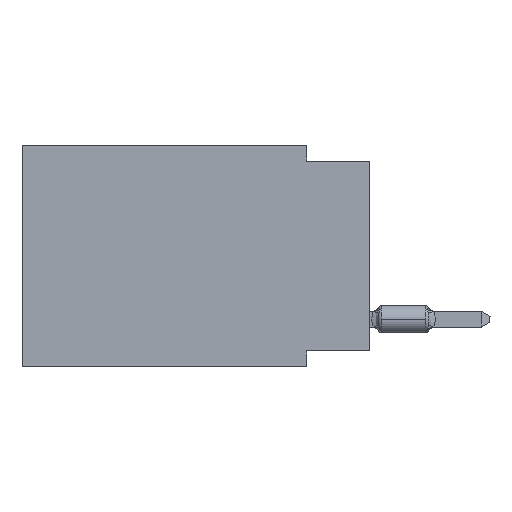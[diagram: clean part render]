
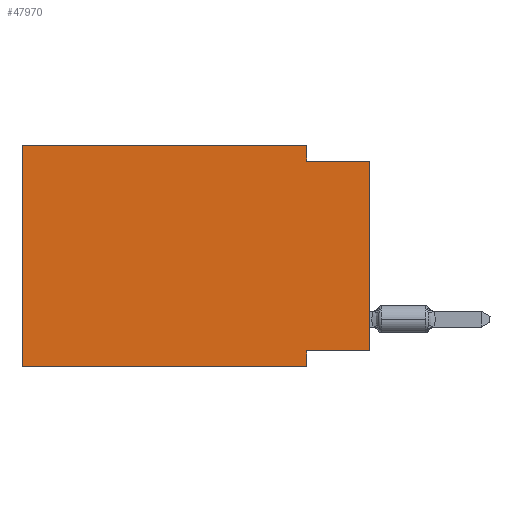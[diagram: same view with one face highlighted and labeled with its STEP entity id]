
A CAD part, left-side view. The second image highlights one B-rep face of the part: STEP entity #47970.
In plain terms, the highlighted planar face has unit normal (-1, 0, 0).
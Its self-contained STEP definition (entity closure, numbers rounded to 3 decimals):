
#74 = EDGE_CURVE ( 'NONE', #14920, #34732, #71550, .T. ) ;
#861 = CARTESIAN_POINT ( 'NONE',  ( 0., 0., -8.255 ) ) ;
#1129 = VERTEX_POINT ( 'NONE', #37625 ) ;
#1969 = LINE ( 'NONE', #44744, #39972 ) ;
#2510 = VERTEX_POINT ( 'NONE', #58885 ) ;
#4873 = LINE ( 'NONE', #11194, #41778 ) ;
#4916 = ORIENTED_EDGE ( 'NONE', *, *, #40327, .F. ) ;
#5290 = ORIENTED_EDGE ( 'NONE', *, *, #49267, .F. ) ;
#5528 = VECTOR ( 'NONE', #20194, 1000. ) ;
#7954 = VECTOR ( 'NONE', #27954, 1000. ) ;
#8227 = DIRECTION ( 'NONE',  ( 0., 0., -1. ) ) ;
#8551 = EDGE_CURVE ( 'NONE', #14920, #77421, #48816, .T. ) ;
#10298 = VECTOR ( 'NONE', #41719, 1000. ) ;
#11194 = CARTESIAN_POINT ( 'NONE',  ( 0., 0., -0.635 ) ) ;
#11829 = DIRECTION ( 'NONE',  ( 0., 0., -1. ) ) ;
#12386 = VERTEX_POINT ( 'NONE', #71640 ) ;
#14219 = LINE ( 'NONE', #50292, #5528 ) ;
#14920 = VERTEX_POINT ( 'NONE', #39695 ) ;
#15002 = ORIENTED_EDGE ( 'NONE', *, *, #8551, .F. ) ;
#16482 = CARTESIAN_POINT ( 'NONE',  ( 0., 2.54, -8.255 ) ) ;
#17542 = ORIENTED_EDGE ( 'NONE', *, *, #74, .T. ) ;
#18570 = PLANE ( 'NONE',  #43942 ) ;
#19170 = ORIENTED_EDGE ( 'NONE', *, *, #73306, .F. ) ;
#20041 = VECTOR ( 'NONE', #8227, 1000. ) ;
#20194 = DIRECTION ( 'NONE',  ( 0., 0., 1. ) ) ;
#20513 = CARTESIAN_POINT ( 'NONE',  ( 0., 2.54, 0. ) ) ;
#21476 = ORIENTED_EDGE ( 'NONE', *, *, #29400, .F. ) ;
#25407 = CARTESIAN_POINT ( 'NONE',  ( 0., 13.97, -8.89 ) ) ;
#27954 = DIRECTION ( 'NONE',  ( 0., 0., 1. ) ) ;
#29272 = DIRECTION ( 'NONE',  ( 1., 0., 0. ) ) ;
#29400 = EDGE_CURVE ( 'NONE', #1129, #34732, #4873, .T. ) ;
#34732 = VERTEX_POINT ( 'NONE', #48716 ) ;
#37157 = LINE ( 'NONE', #20513, #20041 ) ;
#37416 = VERTEX_POINT ( 'NONE', #25407 ) ;
#37551 = LINE ( 'NONE', #56172, #40257 ) ;
#37625 = CARTESIAN_POINT ( 'NONE',  ( 0., 2.54, -0.635 ) ) ;
#39207 = DIRECTION ( 'NONE',  ( 0., -1., 0. ) ) ;
#39381 = ORIENTED_EDGE ( 'NONE', *, *, #46303, .F. ) ;
#39695 = CARTESIAN_POINT ( 'NONE',  ( 0., 0., -8.255 ) ) ;
#39972 = VECTOR ( 'NONE', #63002, 1000. ) ;
#40257 = VECTOR ( 'NONE', #61752, 1000. ) ;
#40327 = EDGE_CURVE ( 'NONE', #2510, #1129, #37157, .T. ) ;
#41719 = DIRECTION ( 'NONE',  ( 0., 1., 0. ) ) ;
#41778 = VECTOR ( 'NONE', #59547, 1000. ) ;
#41809 = CARTESIAN_POINT ( 'NONE',  ( 0., 0., 0. ) ) ;
#42128 = CARTESIAN_POINT ( 'NONE',  ( 0., 13.97, 0. ) ) ;
#43942 = AXIS2_PLACEMENT_3D ( 'NONE', #47899, #29272, #11829 ) ;
#44744 = CARTESIAN_POINT ( 'NONE',  ( 0., 13.97, 0. ) ) ;
#46303 = EDGE_CURVE ( 'NONE', #53779, #2510, #1969, .T. ) ;
#47899 = CARTESIAN_POINT ( 'NONE',  ( 0., 13.97, 0. ) ) ;
#47970 = ADVANCED_FACE ( 'NONE', ( #78053 ), #18570, .F. ) ;
#48716 = CARTESIAN_POINT ( 'NONE',  ( 0., 0., -0.635 ) ) ;
#48816 = LINE ( 'NONE', #861, #10298 ) ;
#49267 = EDGE_CURVE ( 'NONE', #77421, #12386, #37551, .T. ) ;
#50292 = CARTESIAN_POINT ( 'NONE',  ( 0., 13.97, 0. ) ) ;
#51488 = LINE ( 'NONE', #63799, #66362 ) ;
#53779 = VERTEX_POINT ( 'NONE', #42128 ) ;
#55515 = EDGE_CURVE ( 'NONE', #37416, #12386, #51488, .T. ) ;
#56172 = CARTESIAN_POINT ( 'NONE',  ( 0., 2.54, -8.89 ) ) ;
#58641 = EDGE_LOOP ( 'NONE', ( #17542, #21476, #4916, #39381, #19170, #66810, #5290, #15002 ) ) ;
#58885 = CARTESIAN_POINT ( 'NONE',  ( 0., 2.54, 0. ) ) ;
#59547 = DIRECTION ( 'NONE',  ( 0., -1., 0. ) ) ;
#61752 = DIRECTION ( 'NONE',  ( 0., 0., -1. ) ) ;
#63002 = DIRECTION ( 'NONE',  ( 0., -1., 0. ) ) ;
#63799 = CARTESIAN_POINT ( 'NONE',  ( 0., 13.97, -8.89 ) ) ;
#66362 = VECTOR ( 'NONE', #39207, 1000. ) ;
#66810 = ORIENTED_EDGE ( 'NONE', *, *, #55515, .T. ) ;
#71550 = LINE ( 'NONE', #41809, #7954 ) ;
#71640 = CARTESIAN_POINT ( 'NONE',  ( 0., 2.54, -8.89 ) ) ;
#73306 = EDGE_CURVE ( 'NONE', #37416, #53779, #14219, .T. ) ;
#77421 = VERTEX_POINT ( 'NONE', #16482 ) ;
#78053 = FACE_OUTER_BOUND ( 'NONE', #58641, .T. ) ;
